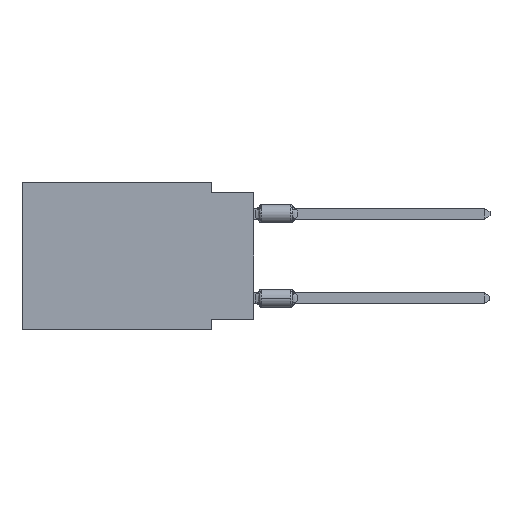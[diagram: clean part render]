
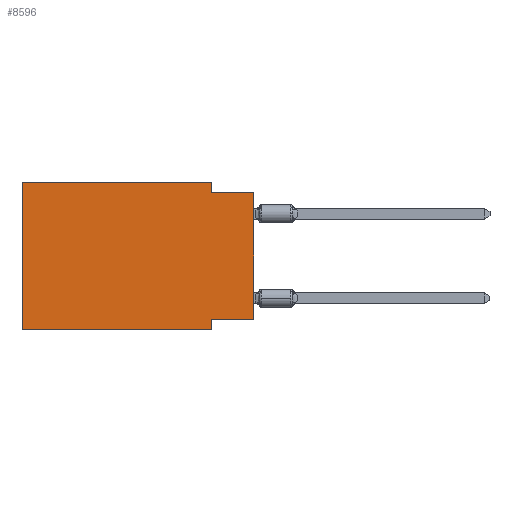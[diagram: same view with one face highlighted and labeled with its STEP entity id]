
A CAD part, left-side view. The second image highlights one B-rep face of the part: STEP entity #8596.
In plain terms, the highlighted planar face has unit normal (-1, 0, 0).
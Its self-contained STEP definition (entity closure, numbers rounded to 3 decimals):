
#658 = LINE ( 'NONE', #21192, #19764 ) ;
#1644 = ORIENTED_EDGE ( 'NONE', *, *, #9977, .F. ) ;
#1794 = VECTOR ( 'NONE', #17956, 1000. ) ;
#1841 = CARTESIAN_POINT ( 'NONE',  ( 0., 0., -0.635 ) ) ;
#1945 = VERTEX_POINT ( 'NONE', #14237 ) ;
#2285 = EDGE_CURVE ( 'NONE', #16173, #16942, #3318, .T. ) ;
#2310 = VECTOR ( 'NONE', #7203, 1000. ) ;
#2533 = VERTEX_POINT ( 'NONE', #4985 ) ;
#2918 = AXIS2_PLACEMENT_3D ( 'NONE', #11840, #30816, #27293 ) ;
#3318 = LINE ( 'NONE', #18578, #22072 ) ;
#4985 = CARTESIAN_POINT ( 'NONE',  ( 0., 2.54, -8.89 ) ) ;
#5216 = DIRECTION ( 'NONE',  ( 0., 0., -1. ) ) ;
#5661 = CARTESIAN_POINT ( 'NONE',  ( 0., 13.97, 0. ) ) ;
#6589 = FACE_OUTER_BOUND ( 'NONE', #29089, .T. ) ;
#7203 = DIRECTION ( 'NONE',  ( 0., -1., 0. ) ) ;
#7872 = LINE ( 'NONE', #15504, #8510 ) ;
#8510 = VECTOR ( 'NONE', #23495, 1000. ) ;
#8596 = ADVANCED_FACE ( 'NONE', ( #6589 ), #30007, .F. ) ;
#9576 = LINE ( 'NONE', #22470, #11549 ) ;
#9588 = ORIENTED_EDGE ( 'NONE', *, *, #12394, .F. ) ;
#9797 = LINE ( 'NONE', #28457, #29556 ) ;
#9977 = EDGE_CURVE ( 'NONE', #14803, #21623, #33421, .T. ) ;
#11549 = VECTOR ( 'NONE', #24355, 1000. ) ;
#11840 = CARTESIAN_POINT ( 'NONE',  ( 0., 13.97, 0. ) ) ;
#12394 = EDGE_CURVE ( 'NONE', #20072, #14803, #18538, .T. ) ;
#12827 = CARTESIAN_POINT ( 'NONE',  ( 0., 13.97, -8.89 ) ) ;
#13455 = DIRECTION ( 'NONE',  ( 0., 0., 1. ) ) ;
#13493 = DIRECTION ( 'NONE',  ( 0., -1., 0. ) ) ;
#14237 = CARTESIAN_POINT ( 'NONE',  ( 0., 0., -8.255 ) ) ;
#14803 = VERTEX_POINT ( 'NONE', #26291 ) ;
#15504 = CARTESIAN_POINT ( 'NONE',  ( 0., 0., -8.255 ) ) ;
#15715 = ORIENTED_EDGE ( 'NONE', *, *, #29342, .F. ) ;
#16173 = VERTEX_POINT ( 'NONE', #23062 ) ;
#16323 = EDGE_CURVE ( 'NONE', #20072, #2533, #27747, .T. ) ;
#16942 = VERTEX_POINT ( 'NONE', #1841 ) ;
#17189 = VERTEX_POINT ( 'NONE', #31200 ) ;
#17956 = DIRECTION ( 'NONE',  ( 0., -1., 0. ) ) ;
#18538 = LINE ( 'NONE', #5661, #21979 ) ;
#18578 = CARTESIAN_POINT ( 'NONE',  ( 0., 0., -0.635 ) ) ;
#19040 = EDGE_CURVE ( 'NONE', #21623, #16173, #9576, .T. ) ;
#19320 = ORIENTED_EDGE ( 'NONE', *, *, #26280, .F. ) ;
#19764 = VECTOR ( 'NONE', #29494, 1000. ) ;
#20072 = VERTEX_POINT ( 'NONE', #12827 ) ;
#20836 = CARTESIAN_POINT ( 'NONE',  ( 0., 13.97, 0. ) ) ;
#21192 = CARTESIAN_POINT ( 'NONE',  ( 0., 0., 0. ) ) ;
#21623 = VERTEX_POINT ( 'NONE', #31255 ) ;
#21979 = VECTOR ( 'NONE', #13455, 1000. ) ;
#22072 = VECTOR ( 'NONE', #13493, 1000. ) ;
#22470 = CARTESIAN_POINT ( 'NONE',  ( 0., 2.54, 0. ) ) ;
#23062 = CARTESIAN_POINT ( 'NONE',  ( 0., 2.54, -0.635 ) ) ;
#23239 = ORIENTED_EDGE ( 'NONE', *, *, #31555, .T. ) ;
#23495 = DIRECTION ( 'NONE',  ( 0., 1., 0. ) ) ;
#23908 = ORIENTED_EDGE ( 'NONE', *, *, #16323, .T. ) ;
#24294 = ORIENTED_EDGE ( 'NONE', *, *, #19040, .F. ) ;
#24355 = DIRECTION ( 'NONE',  ( 0., 0., -1. ) ) ;
#25204 = CARTESIAN_POINT ( 'NONE',  ( 0., 13.97, -8.89 ) ) ;
#26280 = EDGE_CURVE ( 'NONE', #17189, #2533, #9797, .T. ) ;
#26291 = CARTESIAN_POINT ( 'NONE',  ( 0., 13.97, 0. ) ) ;
#27293 = DIRECTION ( 'NONE',  ( 0., 0., -1. ) ) ;
#27747 = LINE ( 'NONE', #25204, #2310 ) ;
#28457 = CARTESIAN_POINT ( 'NONE',  ( 0., 2.54, -8.89 ) ) ;
#29089 = EDGE_LOOP ( 'NONE', ( #23239, #32622, #24294, #1644, #9588, #23908, #19320, #15715 ) ) ;
#29342 = EDGE_CURVE ( 'NONE', #1945, #17189, #7872, .T. ) ;
#29494 = DIRECTION ( 'NONE',  ( 0., 0., 1. ) ) ;
#29556 = VECTOR ( 'NONE', #5216, 1000. ) ;
#30007 = PLANE ( 'NONE',  #2918 ) ;
#30816 = DIRECTION ( 'NONE',  ( 1., 0., 0. ) ) ;
#31200 = CARTESIAN_POINT ( 'NONE',  ( 0., 2.54, -8.255 ) ) ;
#31255 = CARTESIAN_POINT ( 'NONE',  ( 0., 2.54, 0. ) ) ;
#31555 = EDGE_CURVE ( 'NONE', #1945, #16942, #658, .T. ) ;
#32622 = ORIENTED_EDGE ( 'NONE', *, *, #2285, .F. ) ;
#33421 = LINE ( 'NONE', #20836, #1794 ) ;
